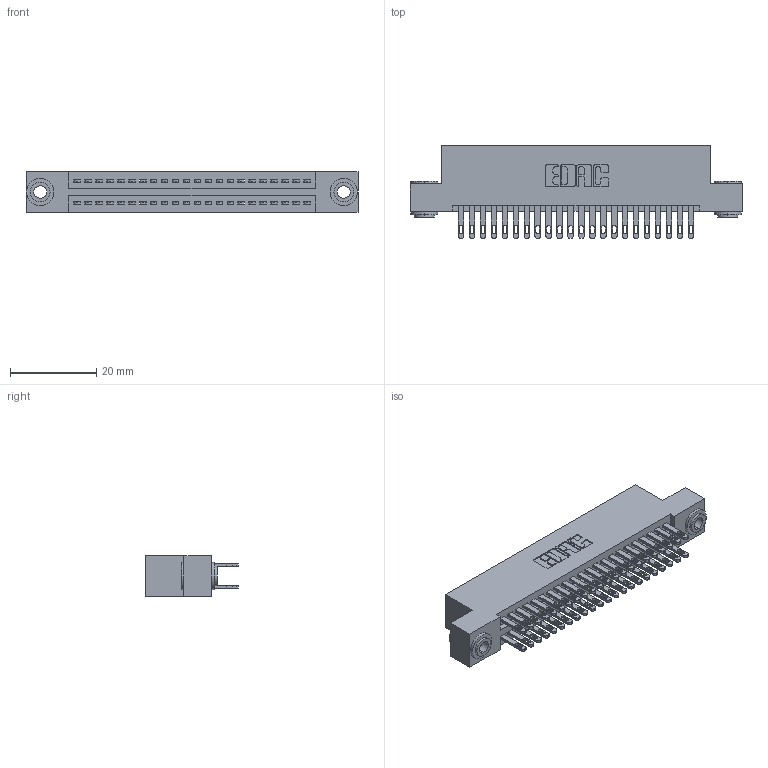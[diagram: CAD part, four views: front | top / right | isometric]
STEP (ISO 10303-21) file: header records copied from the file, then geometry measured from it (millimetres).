
FILE_DESCRIPTION (( 'STEP AP203' ), '1' );
FILE_NAME ('895-044-500-203.STEP', '2020-09-27T02:47:58', ( '' ), ( '' ), 'SwSTEP 2.0', 'SolidWorks 2020', '' );
FILE_SCHEMA (( 'CONFIG_CONTROL_DESIGN' ));
Length unit declared in the file: inch
Products named in the file (4): 845 Part_Flush Mounting Lugs - 0.156 Dia-TH; 895-044-500-203; 345-292-001_345-293-100; 345-250-002_345-250-002-102
Assembly tree (47 placements, depth 2):
  895-044-500-203
    845 Part_Flush Mounting Lugs - 0.156 Dia-TH
    345-292-001_345-293-100  x44
    345-250-002_345-250-002-102  x2
Bounding box: 77.09 x 21.51 x 9.4 mm (x, y, z)
Volume: 7456.7 mm3; surface area: 11288.6 mm2
Topology: 47 solids, 47 shells, 2188 faces, 6621 edges, 4410 vertices
Faces by surface type: plane 1278, cylinder 902, cone 8
Entity records: 20534 total; most frequent: CARTESIAN_POINT 3435, ORIENTED_EDGE 3362, DIRECTION 3087, EDGE_CURVE 1681, LINE 1433, VECTOR 1433, VERTEX_POINT 1118, AXIS2_PLACEMENT_3D 827
